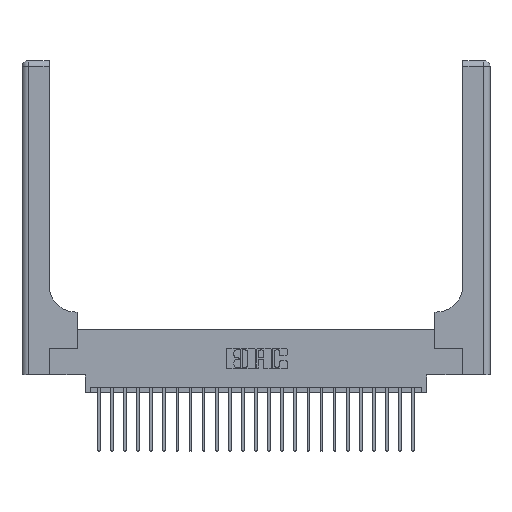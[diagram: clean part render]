
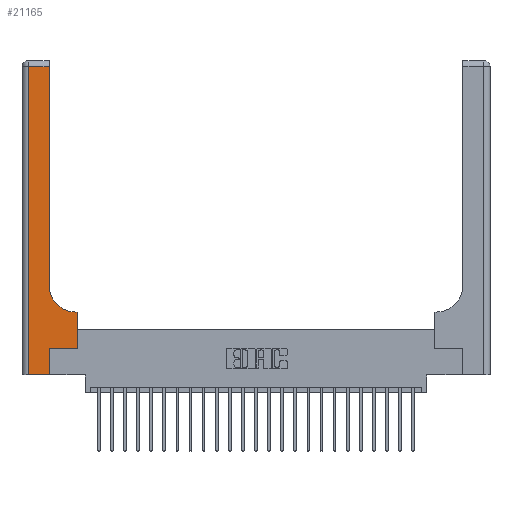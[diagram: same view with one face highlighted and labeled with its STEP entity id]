
A CAD part, top view. The second image highlights one B-rep face of the part: STEP entity #21165.
In plain terms, the highlighted planar face has unit normal (0, 0, 1).
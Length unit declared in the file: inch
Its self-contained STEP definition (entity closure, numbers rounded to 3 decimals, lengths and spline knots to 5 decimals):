
#47 = VERTEX_POINT ( 'NONE', #10124 ) ;
#616 = LINE ( 'NONE', #11970, #23040 ) ;
#804 = CARTESIAN_POINT ( 'NONE',  ( 0., 2.94, 0.37 ) ) ;
#2017 = AXIS2_PLACEMENT_3D ( 'NONE', #17443, #22983, #19316 ) ;
#2028 = DIRECTION ( 'NONE',  ( -1., 0., 0. ) ) ;
#2260 = LINE ( 'NONE', #11410, #19171 ) ;
#2263 = FACE_OUTER_BOUND ( 'NONE', #9476, .T. ) ;
#2881 = ORIENTED_EDGE ( 'NONE', *, *, #2915, .T. ) ;
#2915 = EDGE_CURVE ( 'NONE', #19793, #7352, #616, .T. ) ;
#3654 = DIRECTION ( 'NONE',  ( 1., 0., 0. ) ) ;
#3904 = EDGE_CURVE ( 'NONE', #4993, #12787, #23679, .T. ) ;
#4557 = CARTESIAN_POINT ( 'NONE',  ( 0.265, 0., 0.37 ) ) ;
#4920 = CARTESIAN_POINT ( 'NONE',  ( 0.26, 0.85, 0.37 ) ) ;
#4993 = VERTEX_POINT ( 'NONE', #9968 ) ;
#5198 = CARTESIAN_POINT ( 'NONE',  ( 0.06, 0., 0.37 ) ) ;
#5732 = ORIENTED_EDGE ( 'NONE', *, *, #15586, .T. ) ;
#5760 = CARTESIAN_POINT ( 'NONE',  ( 0.265, 0.25, 0.37 ) ) ;
#6437 = VECTOR ( 'NONE', #20351, 39.37008 ) ;
#7352 = VERTEX_POINT ( 'NONE', #12977 ) ;
#7367 = AXIS2_PLACEMENT_3D ( 'NONE', #17087, #22988, #2028 ) ;
#7576 = ORIENTED_EDGE ( 'NONE', *, *, #3904, .T. ) ;
#7986 = ORIENTED_EDGE ( 'NONE', *, *, #9938, .T. ) ;
#9476 = EDGE_LOOP ( 'NONE', ( #23880, #9785, #7576, #7986, #13227, #13826, #19403, #2881, #5732 ) ) ;
#9785 = ORIENTED_EDGE ( 'NONE', *, *, #21201, .T. ) ;
#9938 = EDGE_CURVE ( 'NONE', #12787, #23781, #13627, .T. ) ;
#9968 = CARTESIAN_POINT ( 'NONE',  ( 0.06, 2.94, 0.37 ) ) ;
#10124 = CARTESIAN_POINT ( 'NONE',  ( 0.265, 0.25, 0.37 ) ) ;
#10268 = VECTOR ( 'NONE', #3654, 39.37008 ) ;
#10284 = LINE ( 'NONE', #804, #14092 ) ;
#10708 = LINE ( 'NONE', #16618, #22198 ) ;
#10874 = EDGE_CURVE ( 'NONE', #47, #20568, #15404, .T. ) ;
#11410 = CARTESIAN_POINT ( 'NONE',  ( 0.26, 3., 0.37 ) ) ;
#11970 = CARTESIAN_POINT ( 'NONE',  ( 0.26, 0.6, 0.37 ) ) ;
#12787 = VERTEX_POINT ( 'NONE', #5198 ) ;
#12977 = CARTESIAN_POINT ( 'NONE',  ( 0.51, 0.6, 0.37 ) ) ;
#13227 = ORIENTED_EDGE ( 'NONE', *, *, #13498, .T. ) ;
#13498 = EDGE_CURVE ( 'NONE', #23781, #47, #21481, .T. ) ;
#13627 = LINE ( 'NONE', #19544, #14837 ) ;
#13826 = ORIENTED_EDGE ( 'NONE', *, *, #10874, .T. ) ;
#14092 = VECTOR ( 'NONE', #18049, 39.37008 ) ;
#14215 = VERTEX_POINT ( 'NONE', #4920 ) ;
#14794 = DIRECTION ( 'NONE',  ( 0., 1., 0. ) ) ;
#14837 = VECTOR ( 'NONE', #23082, 39.37008 ) ;
#15404 = LINE ( 'NONE', #5760, #10268 ) ;
#15586 = EDGE_CURVE ( 'NONE', #7352, #14215, #21707, .T. ) ;
#15755 = VERTEX_POINT ( 'NONE', #16529 ) ;
#16166 = EDGE_CURVE ( 'NONE', #20568, #19793, #10708, .T. ) ;
#16529 = CARTESIAN_POINT ( 'NONE',  ( 0.26, 2.94, 0.37 ) ) ;
#16618 = CARTESIAN_POINT ( 'NONE',  ( 0.528, 0.25, 0.37 ) ) ;
#17087 = CARTESIAN_POINT ( 'NONE',  ( 0., 3., 0.37 ) ) ;
#17443 = CARTESIAN_POINT ( 'NONE',  ( 0.51, 0.85, 0.37 ) ) ;
#17768 = DIRECTION ( 'NONE',  ( 0., 1., 0. ) ) ;
#18049 = DIRECTION ( 'NONE',  ( -1., 0., 0. ) ) ;
#18495 = CARTESIAN_POINT ( 'NONE',  ( 0.528, 0.25, 0.37 ) ) ;
#18945 = PLANE ( 'NONE',  #7367 ) ;
#19171 = VECTOR ( 'NONE', #20909, 39.37008 ) ;
#19316 = DIRECTION ( 'NONE',  ( 1., 0., 0. ) ) ;
#19403 = ORIENTED_EDGE ( 'NONE', *, *, #16166, .T. ) ;
#19544 = CARTESIAN_POINT ( 'NONE',  ( 0., 0., 0.37 ) ) ;
#19793 = VERTEX_POINT ( 'NONE', #23384 ) ;
#20033 = EDGE_CURVE ( 'NONE', #14215, #15755, #2260, .T. ) ;
#20351 = DIRECTION ( 'NONE',  ( 0., -1., 0. ) ) ;
#20568 = VERTEX_POINT ( 'NONE', #18495 ) ;
#20909 = DIRECTION ( 'NONE',  ( 0., 1., 0. ) ) ;
#21165 = ADVANCED_FACE ( 'NONE', ( #2263 ), #18945, .F. ) ;
#21201 = EDGE_CURVE ( 'NONE', #15755, #4993, #10284, .T. ) ;
#21203 = DIRECTION ( 'NONE',  ( -1., 0., 0. ) ) ;
#21481 = LINE ( 'NONE', #4557, #23605 ) ;
#21707 = CIRCLE ( 'NONE', #2017, 0.25 ) ;
#22198 = VECTOR ( 'NONE', #14794, 39.37008 ) ;
#22814 = CARTESIAN_POINT ( 'NONE',  ( 0.265, 0., 0.37 ) ) ;
#22983 = DIRECTION ( 'NONE',  ( 0., 0., -1. ) ) ;
#22988 = DIRECTION ( 'NONE',  ( 0., 0., -1. ) ) ;
#23040 = VECTOR ( 'NONE', #21203, 39.37008 ) ;
#23082 = DIRECTION ( 'NONE',  ( 1., 0., 0. ) ) ;
#23384 = CARTESIAN_POINT ( 'NONE',  ( 0.528, 0.6, 0.37 ) ) ;
#23605 = VECTOR ( 'NONE', #17768, 39.37008 ) ;
#23679 = LINE ( 'NONE', #23918, #6437 ) ;
#23781 = VERTEX_POINT ( 'NONE', #22814 ) ;
#23880 = ORIENTED_EDGE ( 'NONE', *, *, #20033, .T. ) ;
#23918 = CARTESIAN_POINT ( 'NONE',  ( 0.06, 3., 0.37 ) ) ;
